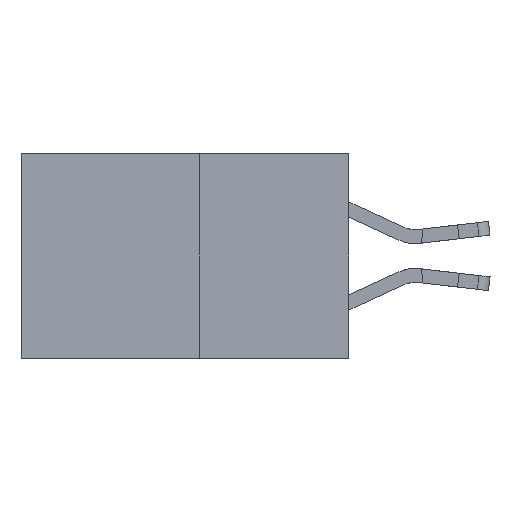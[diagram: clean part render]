
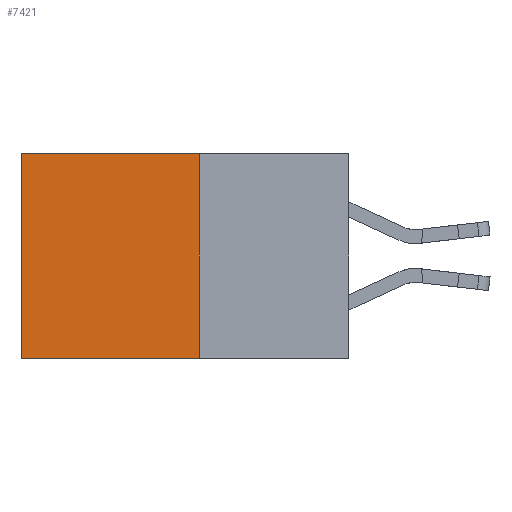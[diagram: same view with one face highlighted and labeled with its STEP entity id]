
A CAD part, left-side view. The second image highlights one B-rep face of the part: STEP entity #7421.
In plain terms, the highlighted planar face has unit normal (-1, 0, 0).
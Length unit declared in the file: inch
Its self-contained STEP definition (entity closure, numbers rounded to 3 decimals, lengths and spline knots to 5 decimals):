
#226 = DIRECTION ( 'NONE',  ( 0., 0., -1. ) ) ;
#626 = VECTOR ( 'NONE', #226, 39.37008 ) ;
#1018 = EDGE_CURVE ( 'NONE', #4812, #3825, #4093, .T. ) ;
#1332 = EDGE_CURVE ( 'NONE', #8951, #3825, #3254, .T. ) ;
#1414 = EDGE_CURVE ( 'NONE', #3202, #8951, #2247, .T. ) ;
#1615 = CARTESIAN_POINT ( 'NONE',  ( 0.277, 0.59, 0. ) ) ;
#2247 = LINE ( 'NONE', #12028, #4771 ) ;
#2619 = DIRECTION ( 'NONE',  ( 0., 1., 0. ) ) ;
#3197 = CARTESIAN_POINT ( 'NONE',  ( 0.277, 0.27, -0.37 ) ) ;
#3202 = VERTEX_POINT ( 'NONE', #12314 ) ;
#3254 = LINE ( 'NONE', #8500, #5833 ) ;
#3495 = LINE ( 'NONE', #6141, #626 ) ;
#3620 = DIRECTION ( 'NONE',  ( 1., 0., 0. ) ) ;
#3734 = ORIENTED_EDGE ( 'NONE', *, *, #4351, .F. ) ;
#3825 = VERTEX_POINT ( 'NONE', #4228 ) ;
#4043 = AXIS2_PLACEMENT_3D ( 'NONE', #7079, #3620, #12958 ) ;
#4093 = LINE ( 'NONE', #13327, #4439 ) ;
#4146 = ORIENTED_EDGE ( 'NONE', *, *, #1018, .F. ) ;
#4228 = CARTESIAN_POINT ( 'NONE',  ( 0.277, 0.59, -0.37 ) ) ;
#4351 = EDGE_CURVE ( 'NONE', #3202, #4812, #3495, .T. ) ;
#4439 = VECTOR ( 'NONE', #6585, 39.37008 ) ;
#4771 = VECTOR ( 'NONE', #2619, 39.37008 ) ;
#4812 = VERTEX_POINT ( 'NONE', #3197 ) ;
#5833 = VECTOR ( 'NONE', #13469, 39.37008 ) ;
#6141 = CARTESIAN_POINT ( 'NONE',  ( 0.277, 0.27, -0.37 ) ) ;
#6381 = FACE_OUTER_BOUND ( 'NONE', #13728, .T. ) ;
#6585 = DIRECTION ( 'NONE',  ( 0., 1., 0. ) ) ;
#7079 = CARTESIAN_POINT ( 'NONE',  ( 0.277, 0.27, -0.37 ) ) ;
#7421 = ADVANCED_FACE ( 'NONE', ( #6381 ), #11905, .F. ) ;
#8500 = CARTESIAN_POINT ( 'NONE',  ( 0.277, 0.59, -0.37 ) ) ;
#8951 = VERTEX_POINT ( 'NONE', #1615 ) ;
#10574 = ORIENTED_EDGE ( 'NONE', *, *, #1332, .T. ) ;
#11905 = PLANE ( 'NONE',  #4043 ) ;
#12028 = CARTESIAN_POINT ( 'NONE',  ( 0.277, 0.27, 0. ) ) ;
#12314 = CARTESIAN_POINT ( 'NONE',  ( 0.277, 0.27, 0. ) ) ;
#12958 = DIRECTION ( 'NONE',  ( 0., 0., -1. ) ) ;
#13327 = CARTESIAN_POINT ( 'NONE',  ( 0.277, 0.27, -0.37 ) ) ;
#13361 = ORIENTED_EDGE ( 'NONE', *, *, #1414, .T. ) ;
#13469 = DIRECTION ( 'NONE',  ( 0., 0., -1. ) ) ;
#13728 = EDGE_LOOP ( 'NONE', ( #10574, #4146, #3734, #13361 ) ) ;
